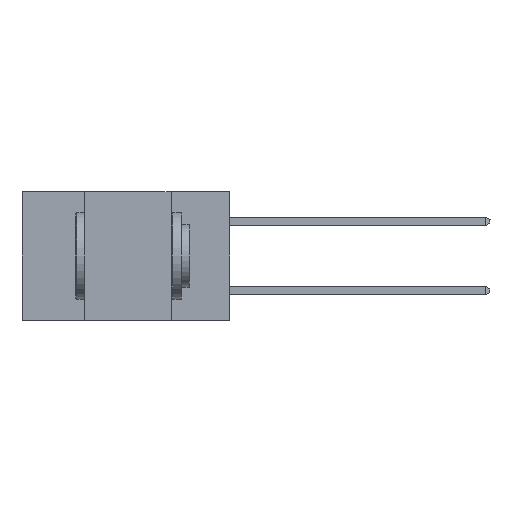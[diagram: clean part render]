
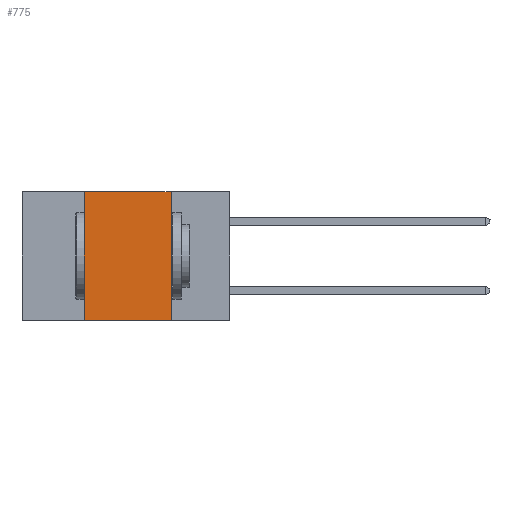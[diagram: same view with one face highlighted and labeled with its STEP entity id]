
A CAD part, left-side view. The second image highlights one B-rep face of the part: STEP entity #775.
In plain terms, the highlighted planar face has unit normal (-1, 0, 0).
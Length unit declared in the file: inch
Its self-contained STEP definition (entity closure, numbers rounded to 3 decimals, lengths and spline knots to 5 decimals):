
#242 = VECTOR ( 'NONE', #7462, 39.37008 ) ;
#775 = ADVANCED_FACE ( 'NONE', ( #3565 ), #2671, .F. ) ;
#839 = VERTEX_POINT ( 'NONE', #2729 ) ;
#1564 = VERTEX_POINT ( 'NONE', #6469 ) ;
#1927 = DIRECTION ( 'NONE',  ( 0., 0., -1. ) ) ;
#2422 = CARTESIAN_POINT ( 'NONE',  ( 0., 0.17, -0.37 ) ) ;
#2671 = PLANE ( 'NONE',  #8570 ) ;
#2729 = CARTESIAN_POINT ( 'NONE',  ( 0., 0.17, 0. ) ) ;
#2935 = CARTESIAN_POINT ( 'NONE',  ( 0., 0.6, -0.37 ) ) ;
#3350 = VECTOR ( 'NONE', #4523, 39.37008 ) ;
#3565 = FACE_OUTER_BOUND ( 'NONE', #5102, .T. ) ;
#3623 = DIRECTION ( 'NONE',  ( 0., 0., 1. ) ) ;
#3679 = CARTESIAN_POINT ( 'NONE',  ( 0., 0.42, -0.37 ) ) ;
#3723 = LINE ( 'NONE', #8311, #8595 ) ;
#3941 = ORIENTED_EDGE ( 'NONE', *, *, #6405, .F. ) ;
#3983 = VERTEX_POINT ( 'NONE', #8142 ) ;
#4045 = CARTESIAN_POINT ( 'NONE',  ( 0., 0.42, -0.37 ) ) ;
#4523 = DIRECTION ( 'NONE',  ( 0., 0., -1. ) ) ;
#5102 = EDGE_LOOP ( 'NONE', ( #8970, #9290, #3941, #7718 ) ) ;
#5232 = EDGE_CURVE ( 'NONE', #839, #1564, #7553, .T. ) ;
#5304 = EDGE_CURVE ( 'NONE', #3983, #839, #3723, .T. ) ;
#6121 = LINE ( 'NONE', #2935, #242 ) ;
#6405 = EDGE_CURVE ( 'NONE', #8864, #3983, #9043, .T. ) ;
#6469 = CARTESIAN_POINT ( 'NONE',  ( 0., 0.17, -0.37 ) ) ;
#6539 = VECTOR ( 'NONE', #3623, 39.37008 ) ;
#6604 = CARTESIAN_POINT ( 'NONE',  ( 0., 0.6, 0. ) ) ;
#7462 = DIRECTION ( 'NONE',  ( 0., -1., 0. ) ) ;
#7553 = LINE ( 'NONE', #2422, #3350 ) ;
#7606 = DIRECTION ( 'NONE',  ( 0., -1., 0. ) ) ;
#7718 = ORIENTED_EDGE ( 'NONE', *, *, #8964, .T. ) ;
#8142 = CARTESIAN_POINT ( 'NONE',  ( 0., 0.42, 0. ) ) ;
#8152 = DIRECTION ( 'NONE',  ( 1., 0., 0. ) ) ;
#8311 = CARTESIAN_POINT ( 'NONE',  ( 0., 0.6, 0. ) ) ;
#8570 = AXIS2_PLACEMENT_3D ( 'NONE', #6604, #8152, #1927 ) ;
#8595 = VECTOR ( 'NONE', #7606, 39.37008 ) ;
#8864 = VERTEX_POINT ( 'NONE', #4045 ) ;
#8964 = EDGE_CURVE ( 'NONE', #8864, #1564, #6121, .T. ) ;
#8970 = ORIENTED_EDGE ( 'NONE', *, *, #5232, .F. ) ;
#9043 = LINE ( 'NONE', #3679, #6539 ) ;
#9290 = ORIENTED_EDGE ( 'NONE', *, *, #5304, .F. ) ;
